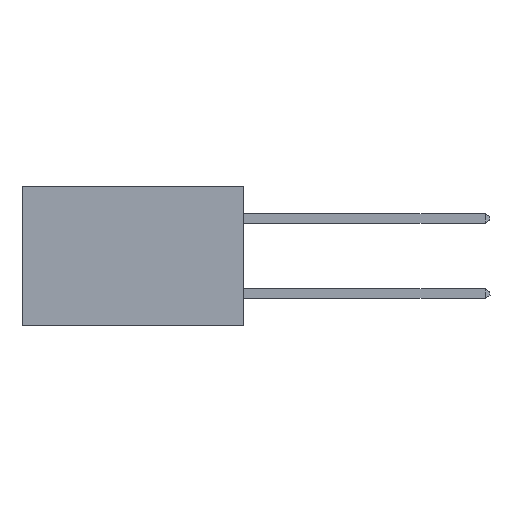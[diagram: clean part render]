
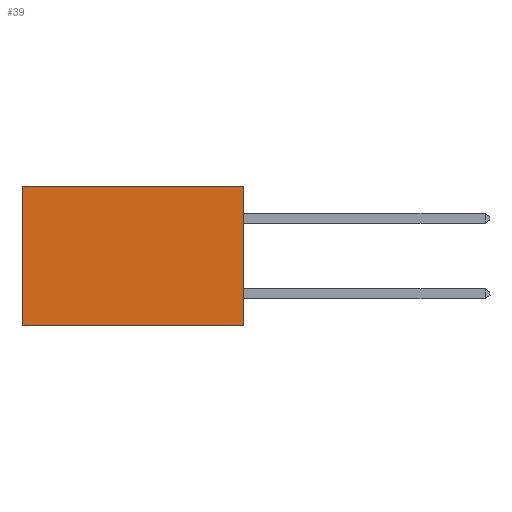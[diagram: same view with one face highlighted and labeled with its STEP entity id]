
A CAD part, left-side view. The second image highlights one B-rep face of the part: STEP entity #39.
In plain terms, the highlighted planar face has unit normal (-1, 0, 0).
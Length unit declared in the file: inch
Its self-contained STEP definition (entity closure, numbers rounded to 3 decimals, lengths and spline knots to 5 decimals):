
#39 = ADVANCED_FACE ( 'NONE', ( #535 ), #155, .F. ) ;
#155 = PLANE ( 'NONE',  #4952 ) ;
#299 = LINE ( 'NONE', #6288, #3481 ) ;
#448 = CARTESIAN_POINT ( 'NONE',  ( 0.277, 0., -0.37 ) ) ;
#535 = FACE_OUTER_BOUND ( 'NONE', #984, .T. ) ;
#957 = VERTEX_POINT ( 'NONE', #448 ) ;
#984 = EDGE_LOOP ( 'NONE', ( #6277, #6658, #7043, #7436 ) ) ;
#2037 = CARTESIAN_POINT ( 'NONE',  ( 0.277, 0.59, -0.37 ) ) ;
#2051 = DIRECTION ( 'NONE',  ( 0., 0., -1. ) ) ;
#2090 = CARTESIAN_POINT ( 'NONE',  ( 0.277, 0.59, -0.37 ) ) ;
#2468 = VECTOR ( 'NONE', #2655, 39.37008 ) ;
#2473 = DIRECTION ( 'NONE',  ( 0., 0., -1. ) ) ;
#2655 = DIRECTION ( 'NONE',  ( 0., 0., -1. ) ) ;
#2672 = LINE ( 'NONE', #2037, #2468 ) ;
#2815 = DIRECTION ( 'NONE',  ( 0., 1., 0. ) ) ;
#2872 = EDGE_CURVE ( 'NONE', #6399, #7854, #4639, .T. ) ;
#3481 = VECTOR ( 'NONE', #6887, 39.37008 ) ;
#4639 = LINE ( 'NONE', #7205, #7772 ) ;
#4952 = AXIS2_PLACEMENT_3D ( 'NONE', #5182, #6430, #2051 ) ;
#5182 = CARTESIAN_POINT ( 'NONE',  ( 0.277, 0., -0.37 ) ) ;
#5364 = VECTOR ( 'NONE', #2473, 39.37008 ) ;
#5603 = CARTESIAN_POINT ( 'NONE',  ( 0.277, 0., -0.37 ) ) ;
#5627 = VERTEX_POINT ( 'NONE', #2090 ) ;
#5765 = LINE ( 'NONE', #5603, #5364 ) ;
#5991 = CARTESIAN_POINT ( 'NONE',  ( 0.277, 0., 0. ) ) ;
#6199 = EDGE_CURVE ( 'NONE', #7854, #5627, #2672, .T. ) ;
#6277 = ORIENTED_EDGE ( 'NONE', *, *, #6199, .T. ) ;
#6288 = CARTESIAN_POINT ( 'NONE',  ( 0.277, 0., -0.37 ) ) ;
#6399 = VERTEX_POINT ( 'NONE', #5991 ) ;
#6430 = DIRECTION ( 'NONE',  ( 1., 0., 0. ) ) ;
#6612 = EDGE_CURVE ( 'NONE', #6399, #957, #5765, .T. ) ;
#6658 = ORIENTED_EDGE ( 'NONE', *, *, #7873, .F. ) ;
#6887 = DIRECTION ( 'NONE',  ( 0., 1., 0. ) ) ;
#7043 = ORIENTED_EDGE ( 'NONE', *, *, #6612, .F. ) ;
#7205 = CARTESIAN_POINT ( 'NONE',  ( 0.277, 0., 0. ) ) ;
#7436 = ORIENTED_EDGE ( 'NONE', *, *, #2872, .T. ) ;
#7772 = VECTOR ( 'NONE', #2815, 39.37008 ) ;
#7854 = VERTEX_POINT ( 'NONE', #8124 ) ;
#7873 = EDGE_CURVE ( 'NONE', #957, #5627, #299, .T. ) ;
#8124 = CARTESIAN_POINT ( 'NONE',  ( 0.277, 0.59, 0. ) ) ;
